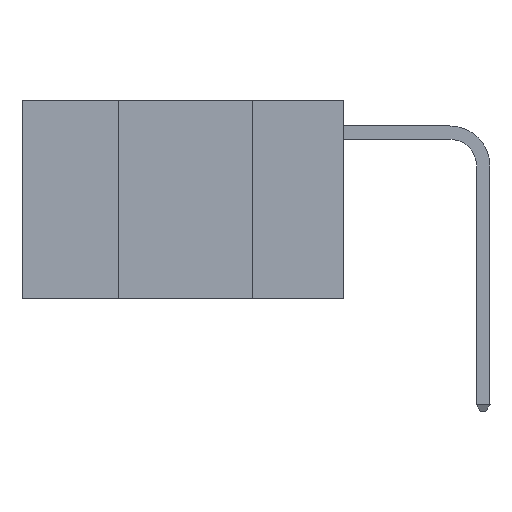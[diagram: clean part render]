
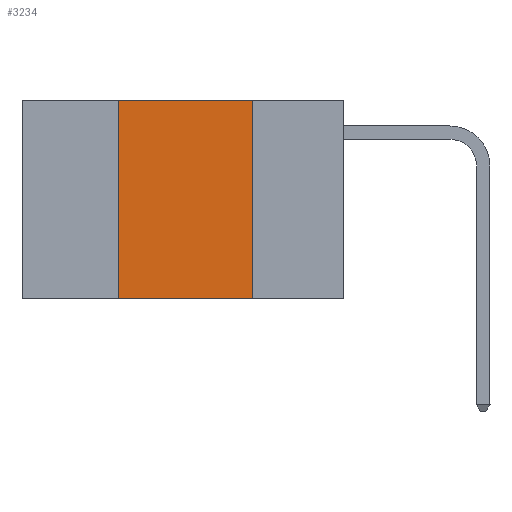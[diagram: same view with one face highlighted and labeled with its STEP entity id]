
A CAD part, left-side view. The second image highlights one B-rep face of the part: STEP entity #3234.
In plain terms, the highlighted planar face has unit normal (-1, 0, 0).
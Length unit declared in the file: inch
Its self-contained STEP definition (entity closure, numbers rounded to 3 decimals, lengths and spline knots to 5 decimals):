
#607 = ORIENTED_EDGE ( 'NONE', *, *, #14547, .T. ) ;
#1245 = VECTOR ( 'NONE', #13614, 39.37008 ) ;
#1877 = AXIS2_PLACEMENT_3D ( 'NONE', #14829, #11417, #5033 ) ;
#2276 = VECTOR ( 'NONE', #5458, 39.37008 ) ;
#2932 = EDGE_CURVE ( 'NONE', #5178, #8452, #10697, .T. ) ;
#3234 = ADVANCED_FACE ( 'NONE', ( #12750 ), #10083, .F. ) ;
#3997 = CARTESIAN_POINT ( 'NONE',  ( 0., 0.17, 0. ) ) ;
#4075 = EDGE_CURVE ( 'NONE', #9032, #5178, #4450, .T. ) ;
#4450 = LINE ( 'NONE', #8981, #6806 ) ;
#4808 = VERTEX_POINT ( 'NONE', #11479 ) ;
#5033 = DIRECTION ( 'NONE',  ( 0., 0., -1. ) ) ;
#5178 = VERTEX_POINT ( 'NONE', #3997 ) ;
#5458 = DIRECTION ( 'NONE',  ( 0., 0., 1. ) ) ;
#6102 = CARTESIAN_POINT ( 'NONE',  ( 0., 0.42, 0. ) ) ;
#6617 = ORIENTED_EDGE ( 'NONE', *, *, #2932, .F. ) ;
#6806 = VECTOR ( 'NONE', #7164, 39.37008 ) ;
#7164 = DIRECTION ( 'NONE',  ( 0., -1., 0. ) ) ;
#7892 = EDGE_LOOP ( 'NONE', ( #6617, #11161, #13080, #607 ) ) ;
#8452 = VERTEX_POINT ( 'NONE', #13200 ) ;
#8981 = CARTESIAN_POINT ( 'NONE',  ( 0., 0.6, 0. ) ) ;
#9032 = VERTEX_POINT ( 'NONE', #6102 ) ;
#9719 = CARTESIAN_POINT ( 'NONE',  ( 0., 0.6, -0.37 ) ) ;
#10083 = PLANE ( 'NONE',  #1877 ) ;
#10662 = CARTESIAN_POINT ( 'NONE',  ( 0., 0.17, 0. ) ) ;
#10697 = LINE ( 'NONE', #10662, #1245 ) ;
#11161 = ORIENTED_EDGE ( 'NONE', *, *, #4075, .F. ) ;
#11223 = LINE ( 'NONE', #9719, #14327 ) ;
#11303 = EDGE_CURVE ( 'NONE', #4808, #9032, #14806, .T. ) ;
#11417 = DIRECTION ( 'NONE',  ( 1., 0., 0. ) ) ;
#11479 = CARTESIAN_POINT ( 'NONE',  ( 0., 0.42, -0.37 ) ) ;
#12505 = CARTESIAN_POINT ( 'NONE',  ( 0., 0.42, 0. ) ) ;
#12750 = FACE_OUTER_BOUND ( 'NONE', #7892, .T. ) ;
#13080 = ORIENTED_EDGE ( 'NONE', *, *, #11303, .F. ) ;
#13200 = CARTESIAN_POINT ( 'NONE',  ( 0., 0.17, -0.37 ) ) ;
#13614 = DIRECTION ( 'NONE',  ( 0., 0., -1. ) ) ;
#14327 = VECTOR ( 'NONE', #14494, 39.37008 ) ;
#14494 = DIRECTION ( 'NONE',  ( 0., -1., 0. ) ) ;
#14547 = EDGE_CURVE ( 'NONE', #4808, #8452, #11223, .T. ) ;
#14806 = LINE ( 'NONE', #12505, #2276 ) ;
#14829 = CARTESIAN_POINT ( 'NONE',  ( 0., 0.6, 0. ) ) ;
